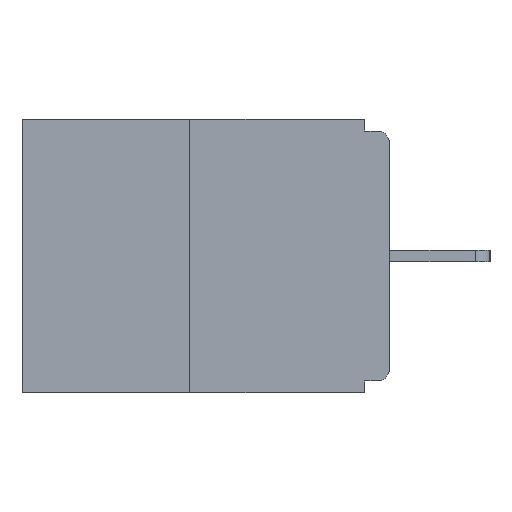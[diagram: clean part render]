
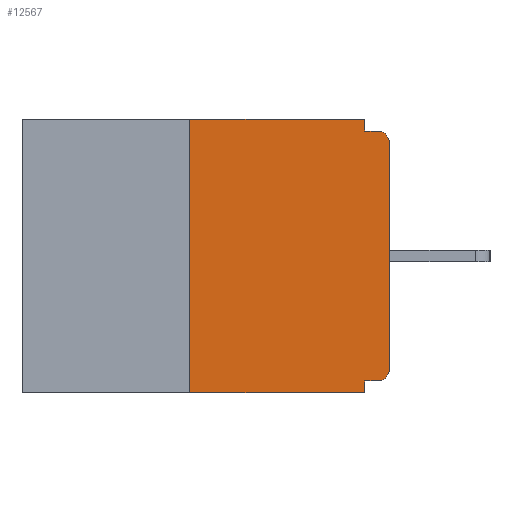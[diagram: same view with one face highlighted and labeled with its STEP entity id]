
A CAD part, left-side view. The second image highlights one B-rep face of the part: STEP entity #12567.
In plain terms, the highlighted planar face has unit normal (-1, 0, 0).
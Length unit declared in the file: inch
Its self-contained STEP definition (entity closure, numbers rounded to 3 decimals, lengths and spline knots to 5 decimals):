
#88 = CARTESIAN_POINT ( 'NONE',  ( 0., 0.031, -0.343 ) ) ;
#201 = VECTOR ( 'NONE', #3999, 39.37008 ) ;
#651 = CARTESIAN_POINT ( 'NONE',  ( 0., 0.25, 0. ) ) ;
#927 = EDGE_CURVE ( 'NONE', #3885, #4252, #8124, .T. ) ;
#938 = VERTEX_POINT ( 'NONE', #3557 ) ;
#954 = ORIENTED_EDGE ( 'NONE', *, *, #6729, .F. ) ;
#1004 = CARTESIAN_POINT ( 'NONE',  ( 0., 0., -0.313 ) ) ;
#1036 = CARTESIAN_POINT ( 'NONE',  ( 0., 0.015, -0.015 ) ) ;
#1216 = AXIS2_PLACEMENT_3D ( 'NONE', #2325, #2938, #3269 ) ;
#1406 = CARTESIAN_POINT ( 'NONE',  ( 0., 0.25, -0.343 ) ) ;
#1507 = PLANE ( 'NONE',  #9063 ) ;
#1552 = CIRCLE ( 'NONE', #1592, 0.015 ) ;
#1592 = AXIS2_PLACEMENT_3D ( 'NONE', #1830, #1817, #2097 ) ;
#1626 = LINE ( 'NONE', #3452, #11914 ) ;
#1639 = ORIENTED_EDGE ( 'NONE', *, *, #927, .F. ) ;
#1782 = VERTEX_POINT ( 'NONE', #9322 ) ;
#1784 = DIRECTION ( 'NONE',  ( 0., -1., 0. ) ) ;
#1817 = DIRECTION ( 'NONE',  ( -1., 0., 0. ) ) ;
#1830 = CARTESIAN_POINT ( 'NONE',  ( 0., 0.015, -0.313 ) ) ;
#2097 = DIRECTION ( 'NONE',  ( 0., 0., -1. ) ) ;
#2125 = DIRECTION ( 'NONE',  ( 0., -1., 0. ) ) ;
#2144 = LINE ( 'NONE', #6374, #12384 ) ;
#2152 = EDGE_LOOP ( 'NONE', ( #2803, #8190, #5926, #11034, #954, #3838, #11621, #11928, #1639, #4526 ) ) ;
#2325 = CARTESIAN_POINT ( 'NONE',  ( 0., 0.015, -0.03 ) ) ;
#2382 = LINE ( 'NONE', #4980, #10313 ) ;
#2404 = CARTESIAN_POINT ( 'NONE',  ( 0., 0.46, -0.343 ) ) ;
#2488 = EDGE_CURVE ( 'NONE', #8280, #1782, #2144, .T. ) ;
#2601 = DIRECTION ( 'NONE',  ( 0., 0., -1. ) ) ;
#2803 = ORIENTED_EDGE ( 'NONE', *, *, #9255, .F. ) ;
#2938 = DIRECTION ( 'NONE',  ( -1., 0., 0. ) ) ;
#3269 = DIRECTION ( 'NONE',  ( 0., 0., -1. ) ) ;
#3452 = CARTESIAN_POINT ( 'NONE',  ( 0., 0.031, 0. ) ) ;
#3557 = CARTESIAN_POINT ( 'NONE',  ( 0., 0.031, 0. ) ) ;
#3838 = ORIENTED_EDGE ( 'NONE', *, *, #5512, .T. ) ;
#3885 = VERTEX_POINT ( 'NONE', #9078 ) ;
#3999 = DIRECTION ( 'NONE',  ( 0., -1., 0. ) ) ;
#4142 = CARTESIAN_POINT ( 'NONE',  ( 0., 0., -0.015 ) ) ;
#4237 = CARTESIAN_POINT ( 'NONE',  ( 0., 0.031, -0.343 ) ) ;
#4252 = VERTEX_POINT ( 'NONE', #1036 ) ;
#4309 = EDGE_CURVE ( 'NONE', #9532, #5402, #7844, .T. ) ;
#4384 = EDGE_CURVE ( 'NONE', #1782, #4252, #12035, .T. ) ;
#4432 = VECTOR ( 'NONE', #2125, 39.37008 ) ;
#4526 = ORIENTED_EDGE ( 'NONE', *, *, #10859, .F. ) ;
#4971 = DIRECTION ( 'NONE',  ( 0., 1., 0. ) ) ;
#4980 = CARTESIAN_POINT ( 'NONE',  ( 0., 0., -0.328 ) ) ;
#5125 = DIRECTION ( 'NONE',  ( 0., 0., -1. ) ) ;
#5402 = VERTEX_POINT ( 'NONE', #4237 ) ;
#5490 = EDGE_CURVE ( 'NONE', #7219, #5402, #7074, .T. ) ;
#5512 = EDGE_CURVE ( 'NONE', #7678, #8280, #1552, .T. ) ;
#5742 = CARTESIAN_POINT ( 'NONE',  ( 0., 0.46, 0. ) ) ;
#5926 = ORIENTED_EDGE ( 'NONE', *, *, #5490, .T. ) ;
#6246 = VECTOR ( 'NONE', #11463, 39.37008 ) ;
#6374 = CARTESIAN_POINT ( 'NONE',  ( 0., 0., 0. ) ) ;
#6523 = DIRECTION ( 'NONE',  ( 0., 0., -1. ) ) ;
#6729 = EDGE_CURVE ( 'NONE', #7678, #9532, #2382, .T. ) ;
#7074 = LINE ( 'NONE', #2404, #4432 ) ;
#7219 = VERTEX_POINT ( 'NONE', #1406 ) ;
#7678 = VERTEX_POINT ( 'NONE', #10105 ) ;
#7844 = LINE ( 'NONE', #88, #10360 ) ;
#7983 = FACE_OUTER_BOUND ( 'NONE', #2152, .T. ) ;
#8124 = LINE ( 'NONE', #4142, #201 ) ;
#8190 = ORIENTED_EDGE ( 'NONE', *, *, #9739, .F. ) ;
#8280 = VERTEX_POINT ( 'NONE', #1004 ) ;
#8512 = LINE ( 'NONE', #12517, #6246 ) ;
#8637 = DIRECTION ( 'NONE',  ( 1., 0., 0. ) ) ;
#9063 = AXIS2_PLACEMENT_3D ( 'NONE', #5742, #8637, #2601 ) ;
#9078 = CARTESIAN_POINT ( 'NONE',  ( 0., 0.031, -0.015 ) ) ;
#9225 = VERTEX_POINT ( 'NONE', #651 ) ;
#9255 = EDGE_CURVE ( 'NONE', #9225, #938, #12102, .T. ) ;
#9304 = CARTESIAN_POINT ( 'NONE',  ( 0., 0.031, -0.328 ) ) ;
#9322 = CARTESIAN_POINT ( 'NONE',  ( 0., 0., -0.03 ) ) ;
#9532 = VERTEX_POINT ( 'NONE', #9304 ) ;
#9739 = EDGE_CURVE ( 'NONE', #7219, #9225, #8512, .T. ) ;
#10105 = CARTESIAN_POINT ( 'NONE',  ( 0., 0.015, -0.328 ) ) ;
#10313 = VECTOR ( 'NONE', #4971, 39.37008 ) ;
#10360 = VECTOR ( 'NONE', #5125, 39.37008 ) ;
#10859 = EDGE_CURVE ( 'NONE', #938, #3885, #1626, .T. ) ;
#11034 = ORIENTED_EDGE ( 'NONE', *, *, #4309, .F. ) ;
#11463 = DIRECTION ( 'NONE',  ( 0., 0., 1. ) ) ;
#11621 = ORIENTED_EDGE ( 'NONE', *, *, #2488, .T. ) ;
#11717 = CARTESIAN_POINT ( 'NONE',  ( 0., 0.46, 0. ) ) ;
#11792 = VECTOR ( 'NONE', #1784, 39.37008 ) ;
#11914 = VECTOR ( 'NONE', #6523, 39.37008 ) ;
#11928 = ORIENTED_EDGE ( 'NONE', *, *, #4384, .T. ) ;
#12035 = CIRCLE ( 'NONE', #1216, 0.015 ) ;
#12102 = LINE ( 'NONE', #11717, #11792 ) ;
#12227 = DIRECTION ( 'NONE',  ( 0., 0., 1. ) ) ;
#12384 = VECTOR ( 'NONE', #12227, 39.37008 ) ;
#12517 = CARTESIAN_POINT ( 'NONE',  ( 0., 0.25, 0. ) ) ;
#12567 = ADVANCED_FACE ( 'NONE', ( #7983 ), #1507, .F. ) ;
